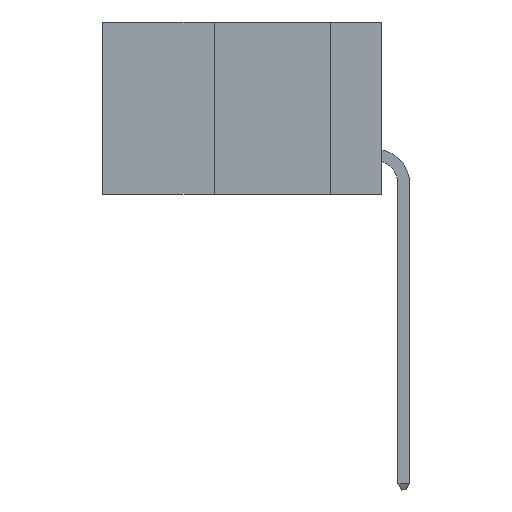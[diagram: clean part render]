
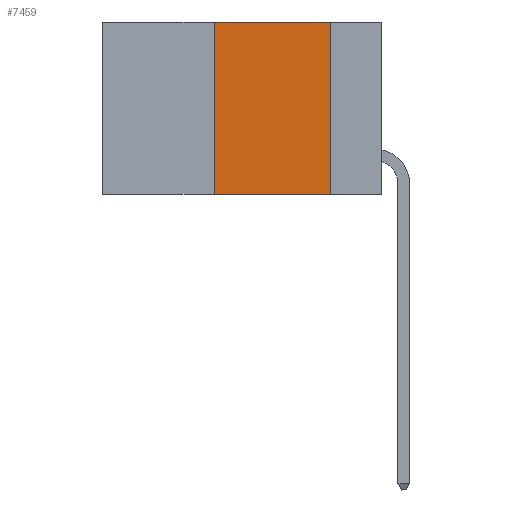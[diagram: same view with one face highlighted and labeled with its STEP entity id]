
A CAD part, left-side view. The second image highlights one B-rep face of the part: STEP entity #7459.
In plain terms, the highlighted planar face has unit normal (-1, 0, 0).
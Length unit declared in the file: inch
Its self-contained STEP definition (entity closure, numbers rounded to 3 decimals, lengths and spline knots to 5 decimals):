
#296 = CARTESIAN_POINT ( 'NONE',  ( 0., 0.11, -0.37 ) ) ;
#662 = DIRECTION ( 'NONE',  ( 1., 0., 0. ) ) ;
#2367 = DIRECTION ( 'NONE',  ( 0., 0., -1. ) ) ;
#3204 = VERTEX_POINT ( 'NONE', #296 ) ;
#3229 = CARTESIAN_POINT ( 'NONE',  ( 0., 0.36, 0. ) ) ;
#3317 = DIRECTION ( 'NONE',  ( 0., 0., 1. ) ) ;
#3709 = VECTOR ( 'NONE', #7207, 39.37008 ) ;
#4182 = LINE ( 'NONE', #6537, #11155 ) ;
#5018 = FACE_OUTER_BOUND ( 'NONE', #24453, .T. ) ;
#5091 = VERTEX_POINT ( 'NONE', #21449 ) ;
#5673 = CARTESIAN_POINT ( 'NONE',  ( 0., 0.11, 0. ) ) ;
#6537 = CARTESIAN_POINT ( 'NONE',  ( 0., 0.6, 0. ) ) ;
#7207 = DIRECTION ( 'NONE',  ( 0., -1., 0. ) ) ;
#7345 = VERTEX_POINT ( 'NONE', #15164 ) ;
#7433 = ORIENTED_EDGE ( 'NONE', *, *, #9090, .F. ) ;
#7459 = ADVANCED_FACE ( 'NONE', ( #5018 ), #12208, .F. ) ;
#7681 = ORIENTED_EDGE ( 'NONE', *, *, #24132, .F. ) ;
#9027 = ORIENTED_EDGE ( 'NONE', *, *, #9312, .T. ) ;
#9046 = CARTESIAN_POINT ( 'NONE',  ( 0., 0.6, -0.37 ) ) ;
#9090 = EDGE_CURVE ( 'NONE', #7345, #3204, #18176, .T. ) ;
#9312 = EDGE_CURVE ( 'NONE', #16665, #3204, #19063, .T. ) ;
#9396 = DIRECTION ( 'NONE',  ( 0., 0., -1. ) ) ;
#11155 = VECTOR ( 'NONE', #18135, 39.37008 ) ;
#12208 = PLANE ( 'NONE',  #20507 ) ;
#12616 = LINE ( 'NONE', #3229, #15610 ) ;
#13800 = CARTESIAN_POINT ( 'NONE',  ( 0., 0.6, 0. ) ) ;
#14044 = ORIENTED_EDGE ( 'NONE', *, *, #18872, .F. ) ;
#15164 = CARTESIAN_POINT ( 'NONE',  ( 0., 0.11, 0. ) ) ;
#15610 = VECTOR ( 'NONE', #3317, 39.37008 ) ;
#16665 = VERTEX_POINT ( 'NONE', #17215 ) ;
#17215 = CARTESIAN_POINT ( 'NONE',  ( 0., 0.36, -0.37 ) ) ;
#18135 = DIRECTION ( 'NONE',  ( 0., -1., 0. ) ) ;
#18176 = LINE ( 'NONE', #5673, #20891 ) ;
#18872 = EDGE_CURVE ( 'NONE', #16665, #5091, #12616, .T. ) ;
#19063 = LINE ( 'NONE', #9046, #3709 ) ;
#20507 = AXIS2_PLACEMENT_3D ( 'NONE', #13800, #662, #2367 ) ;
#20891 = VECTOR ( 'NONE', #9396, 39.37008 ) ;
#21449 = CARTESIAN_POINT ( 'NONE',  ( 0., 0.36, 0. ) ) ;
#24132 = EDGE_CURVE ( 'NONE', #5091, #7345, #4182, .T. ) ;
#24453 = EDGE_LOOP ( 'NONE', ( #7433, #7681, #14044, #9027 ) ) ;
